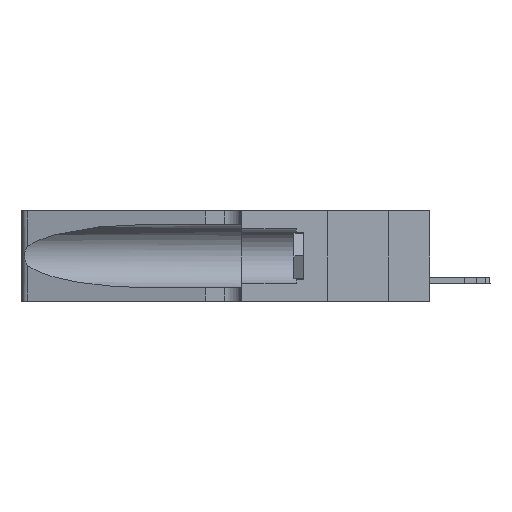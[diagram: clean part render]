
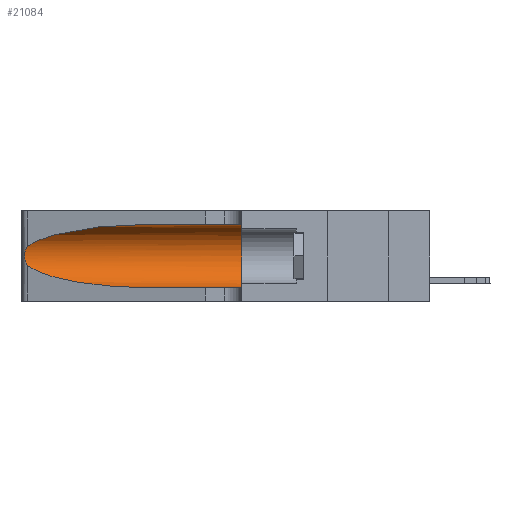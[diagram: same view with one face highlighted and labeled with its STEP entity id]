
A CAD part, left-side view. The second image highlights one B-rep face of the part: STEP entity #21084.
In plain terms, the highlighted cylindrical face has radius 3.308 mm (diameter 6.617 mm), a partial arc.
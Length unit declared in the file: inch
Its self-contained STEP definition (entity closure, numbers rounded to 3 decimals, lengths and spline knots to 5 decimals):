
#500 = EDGE_LOOP ( 'NONE', ( #15376, #29542, #13157, #32809, #16641, #22220 ) ) ;
#954 = CARTESIAN_POINT ( 'NONE',  ( 0.1305, 0.72297, 0.31525 ) ) ;
#1196 = CARTESIAN_POINT ( 'NONE',  ( 0.25789, 1.23486, 0.15765 ) ) ;
#1596 = CARTESIAN_POINT ( 'NONE',  ( 0.25854, 1.2359, 0.20912 ) ) ;
#2546 = CYLINDRICAL_SURFACE ( 'NONE', #29998, 0.13025 ) ;
#2617 = EDGE_CURVE ( 'NONE', #37730, #6104, #4405, .T. ) ;
#4405 = B_SPLINE_CURVE_WITH_KNOTS ( 'NONE', 3,
 ( #10158, #4663, #30925, #33869, #1596, #28225, #16179, #36454, #18763, #21903, #1196, #21753, #24882, #7252 ),
 .UNSPECIFIED., .F., .F.,
 ( 4, 2, 2, 2, 2, 2, 4 ),
 ( 0., 0.00027, 0.00053, 0.00107, 0.0016, 0.00187, 0.00214 ),
 .UNSPECIFIED. ) ;
#4663 = CARTESIAN_POINT ( 'NONE',  ( 0.25555, 1.22994, 0.2215 ) ) ;
#5249 = VECTOR ( 'NONE', #36231, 39.37008 ) ;
#6103 = CARTESIAN_POINT ( 'NONE',  ( 0.1305, 0.35, 0.05475 ) ) ;
#6104 = VERTEX_POINT ( 'NONE', #20709 ) ;
#6649 = CARTESIAN_POINT ( 'NONE',  ( 0.25487, 1.22718, 0.22369 ) ) ;
#6996 = CARTESIAN_POINT ( 'NONE',  ( 0.1305, 1.61858, 0.05475 ) ) ;
#7252 = CARTESIAN_POINT ( 'NONE',  ( 0.25487, 1.22718, 0.14631 ) ) ;
#7336 = CARTESIAN_POINT ( 'NONE',  ( 0.1305, 1.61858, 0.31525 ) ) ;
#9974 = CARTESIAN_POINT ( 'NONE',  ( 0.1305, 0.72297, 0.05475 ) ) ;
#10158 = CARTESIAN_POINT ( 'NONE',  ( 0.25487, 1.22718, 0.22369 ) ) ;
#11347 = DIRECTION ( 'NONE',  ( 0., 0., 1. ) ) ;
#12424 = CARTESIAN_POINT ( 'NONE',  ( 0.1305, 0.35, 0.31525 ) ) ;
#12439 = EDGE_CURVE ( 'NONE', #34688, #22204, #13372, .T. ) ;
#13157 = ORIENTED_EDGE ( 'NONE', *, *, #26574, .T. ) ;
#13199 = EDGE_CURVE ( 'NONE', #33079, #34688, #16027, .T. ) ;
#13372 = CIRCLE ( 'NONE', #25869, 0.13025 ) ;
#15194 =( BOUNDED_CURVE ( )  B_SPLINE_CURVE ( 3, ( #30087, #36398, #18714, #9974 ),
 .UNSPECIFIED., .F., .F. ) 
 B_SPLINE_CURVE_WITH_KNOTS ( ( 4, 4 ),
 ( 3.44316, 4.71239 ),
 .UNSPECIFIED. ) 
 CURVE ( )  GEOMETRIC_REPRESENTATION_ITEM ( )  RATIONAL_B_SPLINE_CURVE ( ( 1., 0.87, 0.87, 1. ) ) 
 REPRESENTATION_ITEM ( '' )  );
#15376 = ORIENTED_EDGE ( 'NONE', *, *, #30848, .T. ) ;
#16027 = LINE ( 'NONE', #7336, #27628 ) ;
#16179 = CARTESIAN_POINT ( 'NONE',  ( 0.26075, 1.23896, 0.19203 ) ) ;
#16641 = ORIENTED_EDGE ( 'NONE', *, *, #12439, .F. ) ;
#17035 = CARTESIAN_POINT ( 'NONE',  ( 0.2373, 1.15595, 0.28018 ) ) ;
#17149 = DIRECTION ( 'NONE',  ( 0., 1., 0. ) ) ;
#18714 = CARTESIAN_POINT ( 'NONE',  ( 0.18966, 0.96281, 0.05475 ) ) ;
#18763 = CARTESIAN_POINT ( 'NONE',  ( 0.26017, 1.23833, 0.17102 ) ) ;
#20227 = CARTESIAN_POINT ( 'NONE',  ( 0.1305, 0.35, 0.185 ) ) ;
#20443 = FACE_OUTER_BOUND ( 'NONE', #500, .T. ) ;
#20709 = CARTESIAN_POINT ( 'NONE',  ( 0.25487, 1.22718, 0.14631 ) ) ;
#21084 = ADVANCED_FACE ( 'NONE', ( #20443 ), #2546, .F. ) ;
#21753 = CARTESIAN_POINT ( 'NONE',  ( 0.25639, 1.23186, 0.15144 ) ) ;
#21799 = LINE ( 'NONE', #6996, #5249 ) ;
#21903 = CARTESIAN_POINT ( 'NONE',  ( 0.25856, 1.23593, 0.16098 ) ) ;
#22204 = VERTEX_POINT ( 'NONE', #6103 ) ;
#22220 = ORIENTED_EDGE ( 'NONE', *, *, #13199, .F. ) ;
#22344 = EDGE_CURVE ( 'NONE', #22765, #22204, #21799, .T. ) ;
#22765 = VERTEX_POINT ( 'NONE', #24058 ) ;
#24058 = CARTESIAN_POINT ( 'NONE',  ( 0.1305, 0.72297, 0.05475 ) ) ;
#24442 = DIRECTION ( 'NONE',  ( 0., -1., 0. ) ) ;
#24882 = CARTESIAN_POINT ( 'NONE',  ( 0.25555, 1.22993, 0.14849 ) ) ;
#25452 = CARTESIAN_POINT ( 'NONE',  ( 0.18966, 0.96281, 0.31525 ) ) ;
#25590 = CARTESIAN_POINT ( 'NONE',  ( 0.25487, 1.22718, 0.22369 ) ) ;
#25869 = AXIS2_PLACEMENT_3D ( 'NONE', #20227, #17149, #11347 ) ;
#26122 =( BOUNDED_CURVE ( )  B_SPLINE_CURVE ( 3, ( #37702, #25452, #17035, #25590 ),
 .UNSPECIFIED., .F., .F. ) 
 B_SPLINE_CURVE_WITH_KNOTS ( ( 4, 4 ),
 ( 1.5708, 2.84003 ),
 .UNSPECIFIED. ) 
 CURVE ( )  GEOMETRIC_REPRESENTATION_ITEM ( )  RATIONAL_B_SPLINE_CURVE ( ( 1., 0.87, 0.87, 1. ) ) 
 REPRESENTATION_ITEM ( '' )  );
#26574 = EDGE_CURVE ( 'NONE', #6104, #22765, #15194, .T. ) ;
#27359 = DIRECTION ( 'NONE',  ( 0., 0., -1. ) ) ;
#27628 = VECTOR ( 'NONE', #24442, 39.37008 ) ;
#28225 = CARTESIAN_POINT ( 'NONE',  ( 0.26018, 1.23835, 0.19895 ) ) ;
#29542 = ORIENTED_EDGE ( 'NONE', *, *, #2617, .T. ) ;
#29998 = AXIS2_PLACEMENT_3D ( 'NONE', #32861, #30051, #27359 ) ;
#30051 = DIRECTION ( 'NONE',  ( 0., -1., 0. ) ) ;
#30087 = CARTESIAN_POINT ( 'NONE',  ( 0.25487, 1.22718, 0.14631 ) ) ;
#30848 = EDGE_CURVE ( 'NONE', #33079, #37730, #26122, .T. ) ;
#30925 = CARTESIAN_POINT ( 'NONE',  ( 0.25639, 1.23184, 0.21858 ) ) ;
#32809 = ORIENTED_EDGE ( 'NONE', *, *, #22344, .T. ) ;
#32861 = CARTESIAN_POINT ( 'NONE',  ( 0.1305, 1.61858, 0.185 ) ) ;
#33079 = VERTEX_POINT ( 'NONE', #954 ) ;
#33869 = CARTESIAN_POINT ( 'NONE',  ( 0.25787, 1.23484, 0.2124 ) ) ;
#34688 = VERTEX_POINT ( 'NONE', #12424 ) ;
#36231 = DIRECTION ( 'NONE',  ( 0., -1., 0. ) ) ;
#36398 = CARTESIAN_POINT ( 'NONE',  ( 0.2373, 1.15595, 0.08982 ) ) ;
#36454 = CARTESIAN_POINT ( 'NONE',  ( 0.26075, 1.23896, 0.178 ) ) ;
#37702 = CARTESIAN_POINT ( 'NONE',  ( 0.1305, 0.72297, 0.31525 ) ) ;
#37730 = VERTEX_POINT ( 'NONE', #6649 ) ;
